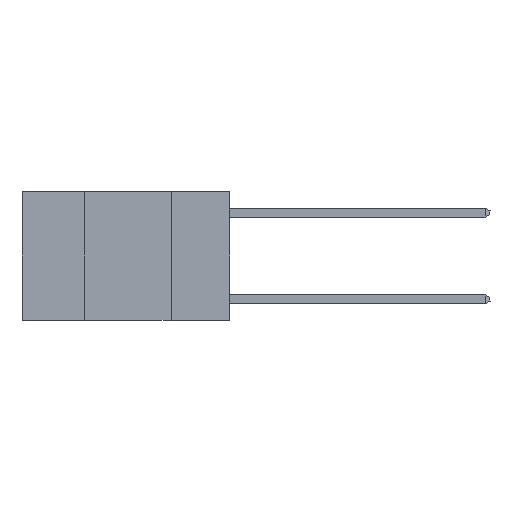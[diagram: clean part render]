
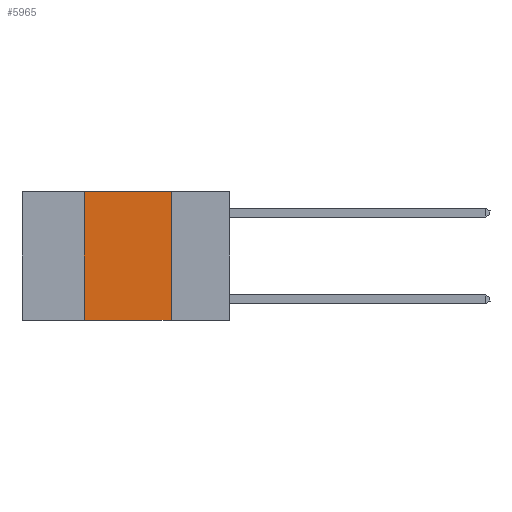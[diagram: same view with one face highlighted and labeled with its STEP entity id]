
A CAD part, left-side view. The second image highlights one B-rep face of the part: STEP entity #5965.
In plain terms, the highlighted planar face has unit normal (-1, 0, 0).
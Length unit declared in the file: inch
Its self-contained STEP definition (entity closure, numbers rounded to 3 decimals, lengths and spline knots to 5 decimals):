
#235 = EDGE_LOOP ( 'NONE', ( #12625, #17560, #19175, #1492 ) ) ;
#830 = VERTEX_POINT ( 'NONE', #20530 ) ;
#1492 = ORIENTED_EDGE ( 'NONE', *, *, #6513, .T. ) ;
#1585 = CARTESIAN_POINT ( 'NONE',  ( 0., 0.17, 0. ) ) ;
#1924 = CARTESIAN_POINT ( 'NONE',  ( 0., 0.17, -0.37 ) ) ;
#1990 = CARTESIAN_POINT ( 'NONE',  ( 0., 0.42, 0. ) ) ;
#2762 = CARTESIAN_POINT ( 'NONE',  ( 0., 0.6, -0.37 ) ) ;
#3779 = EDGE_CURVE ( 'NONE', #830, #9020, #10738, .T. ) ;
#3976 = VECTOR ( 'NONE', #13163, 39.37008 ) ;
#4470 = DIRECTION ( 'NONE',  ( 0., -1., 0. ) ) ;
#4525 = LINE ( 'NONE', #15992, #21030 ) ;
#5657 = CARTESIAN_POINT ( 'NONE',  ( 0., 0.17, 0. ) ) ;
#5965 = ADVANCED_FACE ( 'NONE', ( #15420 ), #6026, .F. ) ;
#6026 = PLANE ( 'NONE',  #9084 ) ;
#6299 = VECTOR ( 'NONE', #15384, 39.37008 ) ;
#6513 = EDGE_CURVE ( 'NONE', #830, #19538, #13111, .T. ) ;
#8951 = LINE ( 'NONE', #1585, #3976 ) ;
#9020 = VERTEX_POINT ( 'NONE', #20590 ) ;
#9084 = AXIS2_PLACEMENT_3D ( 'NONE', #17611, #19329, #9415 ) ;
#9415 = DIRECTION ( 'NONE',  ( 0., 0., -1. ) ) ;
#10533 = VERTEX_POINT ( 'NONE', #5657 ) ;
#10738 = LINE ( 'NONE', #1990, #6299 ) ;
#12625 = ORIENTED_EDGE ( 'NONE', *, *, #18735, .F. ) ;
#13111 = LINE ( 'NONE', #2762, #16994 ) ;
#13152 = EDGE_CURVE ( 'NONE', #9020, #10533, #4525, .T. ) ;
#13163 = DIRECTION ( 'NONE',  ( 0., 0., -1. ) ) ;
#15384 = DIRECTION ( 'NONE',  ( 0., 0., 1. ) ) ;
#15420 = FACE_OUTER_BOUND ( 'NONE', #235, .T. ) ;
#15992 = CARTESIAN_POINT ( 'NONE',  ( 0., 0.6, 0. ) ) ;
#16994 = VECTOR ( 'NONE', #19314, 39.37008 ) ;
#17560 = ORIENTED_EDGE ( 'NONE', *, *, #13152, .F. ) ;
#17611 = CARTESIAN_POINT ( 'NONE',  ( 0., 0.6, 0. ) ) ;
#18735 = EDGE_CURVE ( 'NONE', #10533, #19538, #8951, .T. ) ;
#19175 = ORIENTED_EDGE ( 'NONE', *, *, #3779, .F. ) ;
#19314 = DIRECTION ( 'NONE',  ( 0., -1., 0. ) ) ;
#19329 = DIRECTION ( 'NONE',  ( 1., 0., 0. ) ) ;
#19538 = VERTEX_POINT ( 'NONE', #1924 ) ;
#20530 = CARTESIAN_POINT ( 'NONE',  ( 0., 0.42, -0.37 ) ) ;
#20590 = CARTESIAN_POINT ( 'NONE',  ( 0., 0.42, 0. ) ) ;
#21030 = VECTOR ( 'NONE', #4470, 39.37008 ) ;
